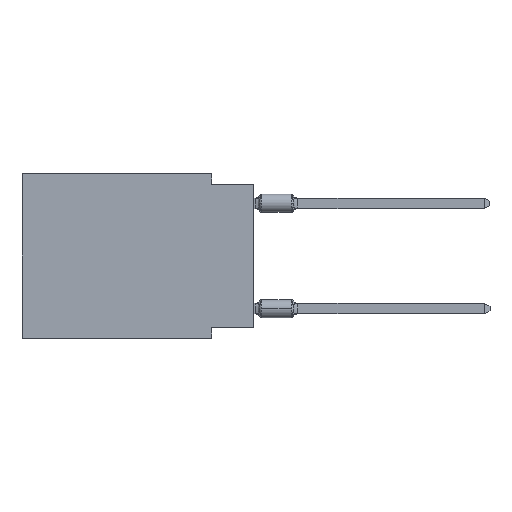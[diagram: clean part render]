
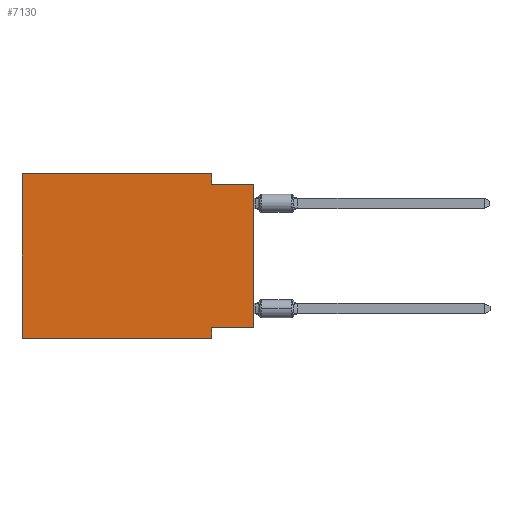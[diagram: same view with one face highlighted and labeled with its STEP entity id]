
A CAD part, left-side view. The second image highlights one B-rep face of the part: STEP entity #7130.
In plain terms, the highlighted planar face has unit normal (-1, 0, 0).
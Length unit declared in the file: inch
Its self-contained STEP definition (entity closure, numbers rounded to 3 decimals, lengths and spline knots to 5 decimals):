
#93 = LINE ( 'NONE', #9200, #2067 ) ;
#118 = EDGE_CURVE ( 'NONE', #2866, #391, #7107, .T. ) ;
#316 = EDGE_CURVE ( 'NONE', #8659, #2611, #2648, .T. ) ;
#391 = VERTEX_POINT ( 'NONE', #12739 ) ;
#913 = DIRECTION ( 'NONE',  ( 0., 0., 1. ) ) ;
#979 = DIRECTION ( 'NONE',  ( 0., 0., -1. ) ) ;
#1476 = ORIENTED_EDGE ( 'NONE', *, *, #3785, .T. ) ;
#1545 = VECTOR ( 'NONE', #979, 39.37008 ) ;
#1605 = AXIS2_PLACEMENT_3D ( 'NONE', #6354, #6165, #9393 ) ;
#1772 = LINE ( 'NONE', #4854, #1545 ) ;
#2013 = VERTEX_POINT ( 'NONE', #10755 ) ;
#2067 = VECTOR ( 'NONE', #10444, 39.37008 ) ;
#2128 = DIRECTION ( 'NONE',  ( 0., 0., 1. ) ) ;
#2181 = VECTOR ( 'NONE', #9731, 39.37008 ) ;
#2414 = CARTESIAN_POINT ( 'NONE',  ( 0., 0.1, -0.025 ) ) ;
#2611 = VERTEX_POINT ( 'NONE', #5091 ) ;
#2617 = DIRECTION ( 'NONE',  ( 0., -1., 0. ) ) ;
#2648 = LINE ( 'NONE', #7567, #2181 ) ;
#2719 = CARTESIAN_POINT ( 'NONE',  ( 0., 0., -0.365 ) ) ;
#2765 = LINE ( 'NONE', #5900, #4470 ) ;
#2866 = VERTEX_POINT ( 'NONE', #3514 ) ;
#3045 = ORIENTED_EDGE ( 'NONE', *, *, #7618, .T. ) ;
#3233 = DIRECTION ( 'NONE',  ( 0., -1., 0. ) ) ;
#3514 = CARTESIAN_POINT ( 'NONE',  ( 0., 0.55, -0.39 ) ) ;
#3728 = EDGE_CURVE ( 'NONE', #2611, #5757, #1772, .T. ) ;
#3785 = EDGE_CURVE ( 'NONE', #8659, #7530, #2765, .T. ) ;
#4243 = ORIENTED_EDGE ( 'NONE', *, *, #4808, .F. ) ;
#4263 = EDGE_CURVE ( 'NONE', #12671, #7530, #8094, .T. ) ;
#4470 = VECTOR ( 'NONE', #913, 39.37008 ) ;
#4643 = LINE ( 'NONE', #7656, #12503 ) ;
#4808 = EDGE_CURVE ( 'NONE', #391, #2013, #6303, .T. ) ;
#4854 = CARTESIAN_POINT ( 'NONE',  ( 0., 0.1, -0.39 ) ) ;
#5091 = CARTESIAN_POINT ( 'NONE',  ( 0., 0.1, -0.365 ) ) ;
#5733 = ORIENTED_EDGE ( 'NONE', *, *, #4263, .F. ) ;
#5757 = VERTEX_POINT ( 'NONE', #9060 ) ;
#5900 = CARTESIAN_POINT ( 'NONE',  ( 0., 0., 0. ) ) ;
#6165 = DIRECTION ( 'NONE',  ( 1., 0., 0. ) ) ;
#6303 = LINE ( 'NONE', #11163, #9320 ) ;
#6314 = DIRECTION ( 'NONE',  ( 0., -1., 0. ) ) ;
#6354 = CARTESIAN_POINT ( 'NONE',  ( 0., 0.55, 0. ) ) ;
#7107 = LINE ( 'NONE', #11111, #12672 ) ;
#7130 = ADVANCED_FACE ( 'NONE', ( #7286 ), #11295, .F. ) ;
#7286 = FACE_OUTER_BOUND ( 'NONE', #12948, .T. ) ;
#7445 = ORIENTED_EDGE ( 'NONE', *, *, #118, .F. ) ;
#7530 = VERTEX_POINT ( 'NONE', #11280 ) ;
#7567 = CARTESIAN_POINT ( 'NONE',  ( 0., 0., -0.365 ) ) ;
#7618 = EDGE_CURVE ( 'NONE', #2866, #5757, #4643, .T. ) ;
#7656 = CARTESIAN_POINT ( 'NONE',  ( 0., 0.55, -0.39 ) ) ;
#8094 = LINE ( 'NONE', #11246, #9516 ) ;
#8659 = VERTEX_POINT ( 'NONE', #2719 ) ;
#8906 = ORIENTED_EDGE ( 'NONE', *, *, #316, .F. ) ;
#9060 = CARTESIAN_POINT ( 'NONE',  ( 0., 0.1, -0.39 ) ) ;
#9200 = CARTESIAN_POINT ( 'NONE',  ( 0., 0.1, 0. ) ) ;
#9320 = VECTOR ( 'NONE', #3233, 39.37008 ) ;
#9393 = DIRECTION ( 'NONE',  ( 0., 0., -1. ) ) ;
#9516 = VECTOR ( 'NONE', #6314, 39.37008 ) ;
#9599 = EDGE_CURVE ( 'NONE', #2013, #12671, #93, .T. ) ;
#9731 = DIRECTION ( 'NONE',  ( 0., 1., 0. ) ) ;
#10285 = ORIENTED_EDGE ( 'NONE', *, *, #3728, .F. ) ;
#10444 = DIRECTION ( 'NONE',  ( 0., 0., -1. ) ) ;
#10755 = CARTESIAN_POINT ( 'NONE',  ( 0., 0.1, 0. ) ) ;
#10855 = ORIENTED_EDGE ( 'NONE', *, *, #9599, .F. ) ;
#11111 = CARTESIAN_POINT ( 'NONE',  ( 0., 0.55, 0. ) ) ;
#11163 = CARTESIAN_POINT ( 'NONE',  ( 0., 0.55, 0. ) ) ;
#11246 = CARTESIAN_POINT ( 'NONE',  ( 0., 0., -0.025 ) ) ;
#11280 = CARTESIAN_POINT ( 'NONE',  ( 0., 0., -0.025 ) ) ;
#11295 = PLANE ( 'NONE',  #1605 ) ;
#12503 = VECTOR ( 'NONE', #2617, 39.37008 ) ;
#12671 = VERTEX_POINT ( 'NONE', #2414 ) ;
#12672 = VECTOR ( 'NONE', #2128, 39.37008 ) ;
#12739 = CARTESIAN_POINT ( 'NONE',  ( 0., 0.55, 0. ) ) ;
#12948 = EDGE_LOOP ( 'NONE', ( #1476, #5733, #10855, #4243, #7445, #3045, #10285, #8906 ) ) ;
